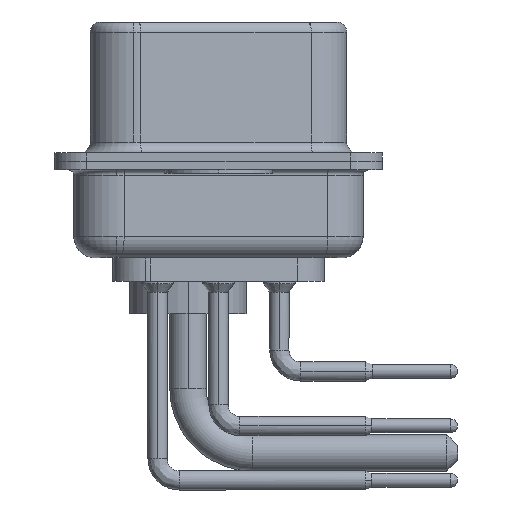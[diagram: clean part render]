
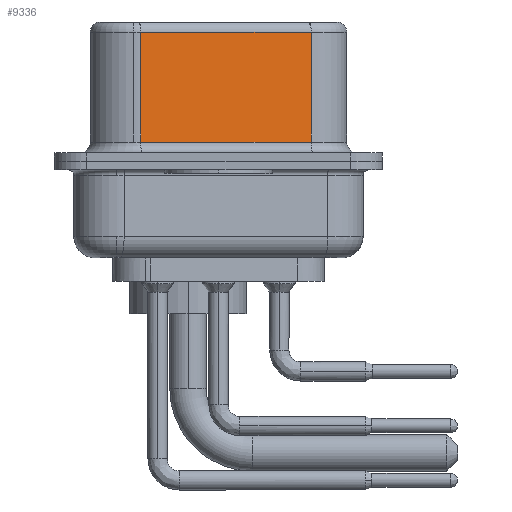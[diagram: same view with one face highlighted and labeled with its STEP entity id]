
A CAD part, left-side view. The second image highlights one B-rep face of the part: STEP entity #9336.
In plain terms, the highlighted planar face has unit normal (-0.985, -0.174, 0).
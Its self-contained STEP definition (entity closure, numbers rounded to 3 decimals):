
#957 = CARTESIAN_POINT ( 'NONE',  ( 5.132, -4.322, 6.02 ) ) ;
#1299 = EDGE_LOOP ( 'NONE', ( #25208, #28853, #14704, #19289 ) ) ;
#1789 = CARTESIAN_POINT ( 'NONE',  ( 3.73, 3.628, 0.9 ) ) ;
#2052 = LINE ( 'NONE', #26902, #25146 ) ;
#5689 = PLANE ( 'NONE',  #6749 ) ;
#6035 = EDGE_CURVE ( 'NONE', #25032, #12264, #33441, .T. ) ;
#6749 = AXIS2_PLACEMENT_3D ( 'NONE', #13997, #24975, #21772 ) ;
#6767 = CARTESIAN_POINT ( 'NONE',  ( 5.132, -4.322, 6.02 ) ) ;
#9336 = ADVANCED_FACE ( 'NONE', ( #27840 ), #5689, .F. ) ;
#11642 = LINE ( 'NONE', #17046, #31294 ) ;
#12264 = VERTEX_POINT ( 'NONE', #18539 ) ;
#13997 = CARTESIAN_POINT ( 'NONE',  ( 5.132, -4.322, 6.52 ) ) ;
#14529 = CARTESIAN_POINT ( 'NONE',  ( 5.132, -4.322, 0.9 ) ) ;
#14704 = ORIENTED_EDGE ( 'NONE', *, *, #24051, .T. ) ;
#16791 = LINE ( 'NONE', #22586, #29935 ) ;
#17046 = CARTESIAN_POINT ( 'NONE',  ( 3.73, 3.628, 6.52 ) ) ;
#18539 = CARTESIAN_POINT ( 'NONE',  ( 3.73, 3.628, 6.02 ) ) ;
#19289 = ORIENTED_EDGE ( 'NONE', *, *, #35264, .T. ) ;
#19949 = DIRECTION ( 'NONE',  ( -0.174, 0.985, 0. ) ) ;
#20441 = VERTEX_POINT ( 'NONE', #14529 ) ;
#21772 = DIRECTION ( 'NONE',  ( -0.174, 0.985, 0. ) ) ;
#22375 = VECTOR ( 'NONE', #19949, 1000. ) ;
#22586 = CARTESIAN_POINT ( 'NONE',  ( 5.132, -4.322, 0.9 ) ) ;
#22659 = DIRECTION ( 'NONE',  ( 0., 0., -1. ) ) ;
#24051 = EDGE_CURVE ( 'NONE', #12264, #25697, #11642, .T. ) ;
#24975 = DIRECTION ( 'NONE',  ( 0.985, 0.174, 0. ) ) ;
#25032 = VERTEX_POINT ( 'NONE', #957 ) ;
#25146 = VECTOR ( 'NONE', #29056, 1000. ) ;
#25208 = ORIENTED_EDGE ( 'NONE', *, *, #31863, .F. ) ;
#25697 = VERTEX_POINT ( 'NONE', #1789 ) ;
#26257 = DIRECTION ( 'NONE',  ( 0.174, -0.985, 0. ) ) ;
#26902 = CARTESIAN_POINT ( 'NONE',  ( 5.132, -4.322, 6.52 ) ) ;
#27840 = FACE_OUTER_BOUND ( 'NONE', #1299, .T. ) ;
#28853 = ORIENTED_EDGE ( 'NONE', *, *, #6035, .T. ) ;
#29056 = DIRECTION ( 'NONE',  ( 0., 0., -1. ) ) ;
#29935 = VECTOR ( 'NONE', #26257, 1000. ) ;
#31294 = VECTOR ( 'NONE', #22659, 1000. ) ;
#31863 = EDGE_CURVE ( 'NONE', #25032, #20441, #2052, .T. ) ;
#33441 = LINE ( 'NONE', #6767, #22375 ) ;
#35264 = EDGE_CURVE ( 'NONE', #25697, #20441, #16791, .T. ) ;
